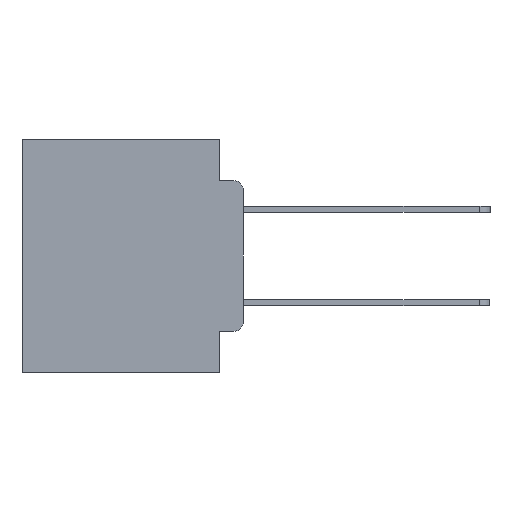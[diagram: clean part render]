
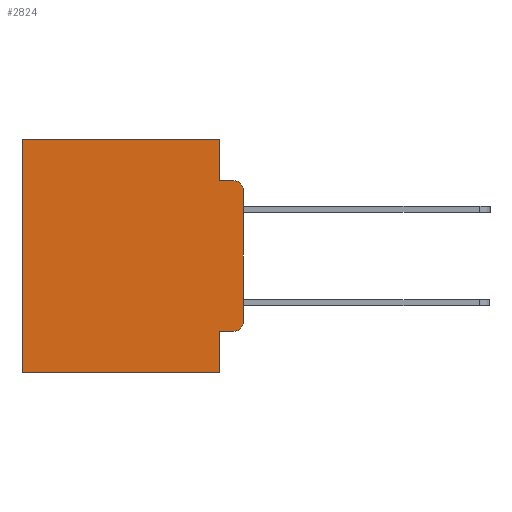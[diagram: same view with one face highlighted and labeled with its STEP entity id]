
A CAD part, left-side view. The second image highlights one B-rep face of the part: STEP entity #2824.
In plain terms, the highlighted planar face has unit normal (-1, 0, 0).
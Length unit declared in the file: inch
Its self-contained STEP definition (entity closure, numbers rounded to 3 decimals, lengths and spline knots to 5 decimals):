
#510 = EDGE_LOOP ( 'NONE', ( #17515, #14663, #18824, #9852, #4299, #5611, #10499, #11762, #22010, #18508 ) ) ;
#965 = DIRECTION ( 'NONE',  ( 0., 1., 0. ) ) ;
#1142 = CARTESIAN_POINT ( 'NONE',  ( 0.298, 0.02, -0.0885 ) ) ;
#1702 = CARTESIAN_POINT ( 'NONE',  ( 0.298, 0., 0. ) ) ;
#2164 = DIRECTION ( 'NONE',  ( 0., -1., 0. ) ) ;
#2578 = LINE ( 'NONE', #13135, #20384 ) ;
#2824 = ADVANCED_FACE ( 'NONE', ( #25329 ), #9003, .F. ) ;
#2870 = DIRECTION ( 'NONE',  ( 1., 0., 0. ) ) ;
#3023 = DIRECTION ( 'NONE',  ( 0., 1., 0. ) ) ;
#4207 = CARTESIAN_POINT ( 'NONE',  ( 0.298, 0.02, -0.1085 ) ) ;
#4236 = LINE ( 'NONE', #15302, #18105 ) ;
#4299 = ORIENTED_EDGE ( 'NONE', *, *, #26301, .T. ) ;
#4318 = DIRECTION ( 'NONE',  ( 0., 0., -1. ) ) ;
#4610 = VECTOR ( 'NONE', #14163, 39.37008 ) ;
#4950 = VECTOR ( 'NONE', #3023, 39.37008 ) ;
#4968 = CARTESIAN_POINT ( 'NONE',  ( 0.298, 0.051, -0.0885 ) ) ;
#4978 = AXIS2_PLACEMENT_3D ( 'NONE', #5289, #19712, #7436 ) ;
#4985 = DIRECTION ( 'NONE',  ( 0., 0., -1. ) ) ;
#5289 = CARTESIAN_POINT ( 'NONE',  ( 0.298, 0.02, -0.3915 ) ) ;
#5476 = CARTESIAN_POINT ( 'NONE',  ( 0.298, 0., -0.3915 ) ) ;
#5611 = ORIENTED_EDGE ( 'NONE', *, *, #13441, .T. ) ;
#5613 = VERTEX_POINT ( 'NONE', #4968 ) ;
#5678 = AXIS2_PLACEMENT_3D ( 'NONE', #9387, #2870, #13022 ) ;
#5742 = VECTOR ( 'NONE', #7963, 39.37008 ) ;
#5832 = CARTESIAN_POINT ( 'NONE',  ( 0.298, 0.051, -0.0885 ) ) ;
#5982 = LINE ( 'NONE', #25801, #21739 ) ;
#6328 = DIRECTION ( 'NONE',  ( 0., 0., -1. ) ) ;
#7086 = EDGE_CURVE ( 'NONE', #19544, #19752, #5982, .T. ) ;
#7436 = DIRECTION ( 'NONE',  ( 0., 0., -1. ) ) ;
#7963 = DIRECTION ( 'NONE',  ( 0., -1., 0. ) ) ;
#9003 = PLANE ( 'NONE',  #5678 ) ;
#9352 = EDGE_CURVE ( 'NONE', #5613, #26367, #16734, .T. ) ;
#9387 = CARTESIAN_POINT ( 'NONE',  ( 0.298, 0., 0. ) ) ;
#9852 = ORIENTED_EDGE ( 'NONE', *, *, #18891, .F. ) ;
#10163 = LINE ( 'NONE', #1702, #4610 ) ;
#10499 = ORIENTED_EDGE ( 'NONE', *, *, #25409, .F. ) ;
#10662 = VERTEX_POINT ( 'NONE', #12283 ) ;
#10717 = EDGE_CURVE ( 'NONE', #12334, #26367, #20812, .T. ) ;
#11762 = ORIENTED_EDGE ( 'NONE', *, *, #12606, .F. ) ;
#12283 = CARTESIAN_POINT ( 'NONE',  ( 0.298, 0.051, -0.5 ) ) ;
#12334 = VERTEX_POINT ( 'NONE', #25769 ) ;
#12606 = EDGE_CURVE ( 'NONE', #19544, #10662, #22622, .T. ) ;
#13022 = DIRECTION ( 'NONE',  ( 0., 0., -1. ) ) ;
#13135 = CARTESIAN_POINT ( 'NONE',  ( 0.298, 0.473, 0. ) ) ;
#13441 = EDGE_CURVE ( 'NONE', #25807, #14304, #2578, .T. ) ;
#13474 = CARTESIAN_POINT ( 'NONE',  ( 0.298, 0.051, 0. ) ) ;
#14163 = DIRECTION ( 'NONE',  ( 0., 0., -1. ) ) ;
#14304 = VERTEX_POINT ( 'NONE', #15282 ) ;
#14663 = ORIENTED_EDGE ( 'NONE', *, *, #10717, .T. ) ;
#15079 = VERTEX_POINT ( 'NONE', #5476 ) ;
#15282 = CARTESIAN_POINT ( 'NONE',  ( 0.298, 0.473, -0.5 ) ) ;
#15302 = CARTESIAN_POINT ( 'NONE',  ( 0.298, 0.051, 0. ) ) ;
#15450 = CARTESIAN_POINT ( 'NONE',  ( 0.298, 0., -0.5 ) ) ;
#16734 = LINE ( 'NONE', #5832, #5742 ) ;
#17203 = VECTOR ( 'NONE', #4318, 39.37008 ) ;
#17503 = CARTESIAN_POINT ( 'NONE',  ( 0.298, 0., 0. ) ) ;
#17515 = ORIENTED_EDGE ( 'NONE', *, *, #25673, .F. ) ;
#18105 = VECTOR ( 'NONE', #4985, 39.37008 ) ;
#18508 = ORIENTED_EDGE ( 'NONE', *, *, #19998, .T. ) ;
#18636 = DIRECTION ( 'NONE',  ( -1., 0., 0. ) ) ;
#18824 = ORIENTED_EDGE ( 'NONE', *, *, #9352, .F. ) ;
#18891 = EDGE_CURVE ( 'NONE', #18964, #5613, #4236, .T. ) ;
#18964 = VERTEX_POINT ( 'NONE', #13474 ) ;
#19544 = VERTEX_POINT ( 'NONE', #25414 ) ;
#19712 = DIRECTION ( 'NONE',  ( -1., 0., 0. ) ) ;
#19752 = VERTEX_POINT ( 'NONE', #21948 ) ;
#19998 = EDGE_CURVE ( 'NONE', #19752, #15079, #20311, .T. ) ;
#20311 = CIRCLE ( 'NONE', #4978, 0.02 ) ;
#20384 = VECTOR ( 'NONE', #25271, 39.37008 ) ;
#20812 = CIRCLE ( 'NONE', #23162, 0.02 ) ;
#21329 = VECTOR ( 'NONE', #965, 39.37008 ) ;
#21739 = VECTOR ( 'NONE', #2164, 39.37008 ) ;
#21948 = CARTESIAN_POINT ( 'NONE',  ( 0.298, 0.02, -0.4115 ) ) ;
#22010 = ORIENTED_EDGE ( 'NONE', *, *, #7086, .T. ) ;
#22622 = LINE ( 'NONE', #22750, #17203 ) ;
#22750 = CARTESIAN_POINT ( 'NONE',  ( 0.298, 0.051, 0. ) ) ;
#23162 = AXIS2_PLACEMENT_3D ( 'NONE', #4207, #18636, #6328 ) ;
#23737 = CARTESIAN_POINT ( 'NONE',  ( 0.298, 0.473, 0. ) ) ;
#25271 = DIRECTION ( 'NONE',  ( 0., 0., -1. ) ) ;
#25329 = FACE_OUTER_BOUND ( 'NONE', #510, .T. ) ;
#25409 = EDGE_CURVE ( 'NONE', #10662, #14304, #26046, .T. ) ;
#25414 = CARTESIAN_POINT ( 'NONE',  ( 0.298, 0.051, -0.4115 ) ) ;
#25673 = EDGE_CURVE ( 'NONE', #12334, #15079, #10163, .T. ) ;
#25769 = CARTESIAN_POINT ( 'NONE',  ( 0.298, 0., -0.1085 ) ) ;
#25801 = CARTESIAN_POINT ( 'NONE',  ( 0.298, 0.051, -0.4115 ) ) ;
#25807 = VERTEX_POINT ( 'NONE', #23737 ) ;
#26046 = LINE ( 'NONE', #15450, #4950 ) ;
#26301 = EDGE_CURVE ( 'NONE', #18964, #25807, #26627, .T. ) ;
#26367 = VERTEX_POINT ( 'NONE', #1142 ) ;
#26627 = LINE ( 'NONE', #17503, #21329 ) ;
